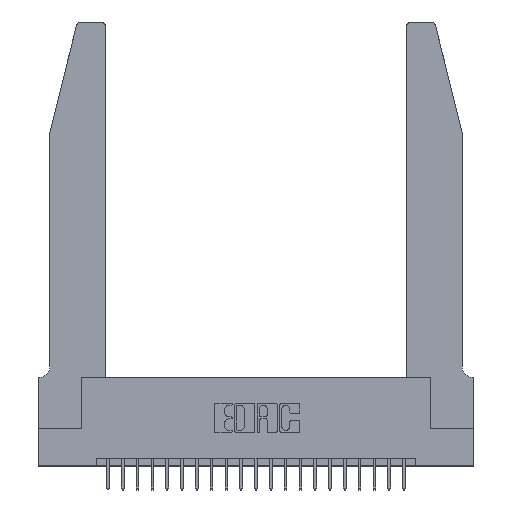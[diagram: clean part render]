
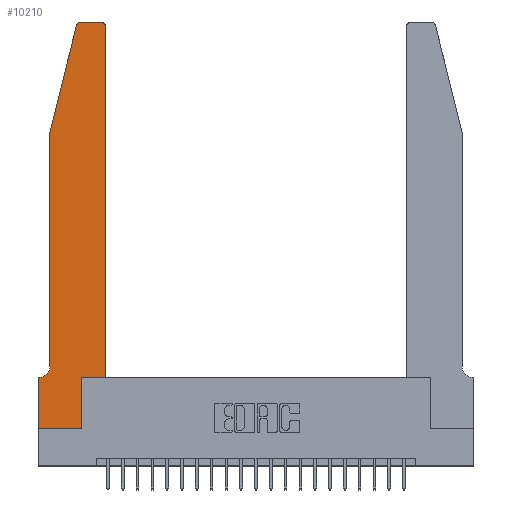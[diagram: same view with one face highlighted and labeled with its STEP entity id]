
A CAD part, top view. The second image highlights one B-rep face of the part: STEP entity #10210.
In plain terms, the highlighted planar face has unit normal (0, 0, 1).
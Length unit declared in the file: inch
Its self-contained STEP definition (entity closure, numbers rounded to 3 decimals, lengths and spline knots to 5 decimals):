
#518 = CARTESIAN_POINT ( 'NONE',  ( 0.4505, 0.35, 0.37 ) ) ;
#969 = ORIENTED_EDGE ( 'NONE', *, *, #10459, .T. ) ;
#1217 = CARTESIAN_POINT ( 'NONE',  ( 0.0755, 2., 0.37 ) ) ;
#1559 = LINE ( 'NONE', #3184, #14602 ) ;
#1598 = CARTESIAN_POINT ( 'NONE',  ( 0.284, 2.75, 0.37 ) ) ;
#2487 = EDGE_CURVE ( 'NONE', #15895, #18629, #21122, .T. ) ;
#2760 = DIRECTION ( 'NONE',  ( 0., -1., 0. ) ) ;
#3184 = CARTESIAN_POINT ( 'NONE',  ( 0.4505, 0.35, 0.37 ) ) ;
#3257 = EDGE_CURVE ( 'NONE', #16590, #14821, #1559, .T. ) ;
#3805 = AXIS2_PLACEMENT_3D ( 'NONE', #23059, #21273, #11658 ) ;
#3820 = VERTEX_POINT ( 'NONE', #13318 ) ;
#4041 = EDGE_CURVE ( 'NONE', #3820, #15895, #5825, .T. ) ;
#4322 = ORIENTED_EDGE ( 'NONE', *, *, #22397, .T. ) ;
#4391 = CIRCLE ( 'NONE', #15009, 0.03 ) ;
#4394 = DIRECTION ( 'NONE',  ( 0., 1., 0. ) ) ;
#4732 = CARTESIAN_POINT ( 'NONE',  ( 0., 0., 0.37 ) ) ;
#4847 = DIRECTION ( 'NONE',  ( -0.239, -0.971, 0. ) ) ;
#4970 = CARTESIAN_POINT ( 'NONE',  ( 0., 0.35, 0.37 ) ) ;
#5180 = ORIENTED_EDGE ( 'NONE', *, *, #2487, .T. ) ;
#5218 = CARTESIAN_POINT ( 'NONE',  ( 0.284, 2.72, 0.37 ) ) ;
#5219 = CARTESIAN_POINT ( 'NONE',  ( 0.2865, 0.35, 0.37 ) ) ;
#5332 = VERTEX_POINT ( 'NONE', #23850 ) ;
#5793 = CIRCLE ( 'NONE', #6472, 0.03 ) ;
#5825 = CIRCLE ( 'NONE', #21263, 0.07 ) ;
#6244 = PLANE ( 'NONE',  #3805 ) ;
#6345 = EDGE_CURVE ( 'NONE', #18629, #5332, #7026, .T. ) ;
#6351 = VERTEX_POINT ( 'NONE', #19138 ) ;
#6428 = EDGE_LOOP ( 'NONE', ( #13984, #10346, #16346, #15535, #10885, #5180, #6851, #6912, #17167, #21293, #969, #4322 ) ) ;
#6472 = AXIS2_PLACEMENT_3D ( 'NONE', #23549, #23231, #12160 ) ;
#6851 = ORIENTED_EDGE ( 'NONE', *, *, #6345, .T. ) ;
#6912 = ORIENTED_EDGE ( 'NONE', *, *, #23955, .T. ) ;
#7026 = LINE ( 'NONE', #11127, #11673 ) ;
#7093 = DIRECTION ( 'NONE',  ( 1., 0., 0. ) ) ;
#7565 = CARTESIAN_POINT ( 'NONE',  ( 0.0755, 0.35, 0.37 ) ) ;
#8272 = EDGE_CURVE ( 'NONE', #18080, #16590, #8691, .T. ) ;
#8353 = VECTOR ( 'NONE', #11817, 39.37008 ) ;
#8691 = LINE ( 'NONE', #14840, #23918 ) ;
#8903 = VERTEX_POINT ( 'NONE', #21593 ) ;
#9242 = VECTOR ( 'NONE', #18430, 39.37008 ) ;
#9879 = CARTESIAN_POINT ( 'NONE',  ( 0.4205, 2.75, 0.37 ) ) ;
#10094 = LINE ( 'NONE', #4732, #9242 ) ;
#10210 = ADVANCED_FACE ( 'NONE', ( #18243 ), #6244, .T. ) ;
#10346 = ORIENTED_EDGE ( 'NONE', *, *, #21312, .T. ) ;
#10459 = EDGE_CURVE ( 'NONE', #14821, #10575, #17035, .T. ) ;
#10575 = VERTEX_POINT ( 'NONE', #20795 ) ;
#10885 = ORIENTED_EDGE ( 'NONE', *, *, #4041, .T. ) ;
#11127 = CARTESIAN_POINT ( 'NONE',  ( 0., 0., 0.37 ) ) ;
#11249 = LINE ( 'NONE', #17401, #8353 ) ;
#11658 = DIRECTION ( 'NONE',  ( 1., 0., 0. ) ) ;
#11673 = VECTOR ( 'NONE', #2760, 39.37008 ) ;
#11817 = DIRECTION ( 'NONE',  ( -1., 0., 0. ) ) ;
#12160 = DIRECTION ( 'NONE',  ( 1., 0., 0. ) ) ;
#12227 = CARTESIAN_POINT ( 'NONE',  ( 0.2865, 0., 0.37 ) ) ;
#13318 = CARTESIAN_POINT ( 'NONE',  ( 0.0755, 0.42, 0.37 ) ) ;
#13984 = ORIENTED_EDGE ( 'NONE', *, *, #15101, .T. ) ;
#14243 = DIRECTION ( 'NONE',  ( 0., 1., 0. ) ) ;
#14574 = DIRECTION ( 'NONE',  ( 0., 0., 1. ) ) ;
#14602 = VECTOR ( 'NONE', #16005, 39.37008 ) ;
#14821 = VERTEX_POINT ( 'NONE', #20120 ) ;
#14840 = CARTESIAN_POINT ( 'NONE',  ( 0.2865, 0.35, 0.37 ) ) ;
#15009 = AXIS2_PLACEMENT_3D ( 'NONE', #5218, #14574, #7093 ) ;
#15010 = DIRECTION ( 'NONE',  ( -1., 0., 0. ) ) ;
#15101 = EDGE_CURVE ( 'NONE', #19637, #21372, #11249, .T. ) ;
#15158 = CARTESIAN_POINT ( 'NONE',  ( 0.0055, 0.42, 0.37 ) ) ;
#15535 = ORIENTED_EDGE ( 'NONE', *, *, #23777, .T. ) ;
#15895 = VERTEX_POINT ( 'NONE', #21940 ) ;
#16005 = DIRECTION ( 'NONE',  ( 1., 0., 0. ) ) ;
#16240 = VECTOR ( 'NONE', #22858, 39.37008 ) ;
#16346 = ORIENTED_EDGE ( 'NONE', *, *, #23406, .T. ) ;
#16590 = VERTEX_POINT ( 'NONE', #5219 ) ;
#17035 = LINE ( 'NONE', #518, #23518 ) ;
#17167 = ORIENTED_EDGE ( 'NONE', *, *, #8272, .T. ) ;
#17230 = DIRECTION ( 'NONE',  ( 0., 0., -1. ) ) ;
#17401 = CARTESIAN_POINT ( 'NONE',  ( 0.2605, 2.75, 0.37 ) ) ;
#17580 = VECTOR ( 'NONE', #21041, 39.37008 ) ;
#18080 = VERTEX_POINT ( 'NONE', #12227 ) ;
#18243 = FACE_OUTER_BOUND ( 'NONE', #6428, .T. ) ;
#18430 = DIRECTION ( 'NONE',  ( 1., 0., 0. ) ) ;
#18629 = VERTEX_POINT ( 'NONE', #4970 ) ;
#19105 = CARTESIAN_POINT ( 'NONE',  ( 0.0755, 2., 0.37 ) ) ;
#19138 = CARTESIAN_POINT ( 'NONE',  ( 0.25487, 2.72718, 0.37 ) ) ;
#19637 = VERTEX_POINT ( 'NONE', #9879 ) ;
#20120 = CARTESIAN_POINT ( 'NONE',  ( 0.4505, 0.35, 0.37 ) ) ;
#20795 = CARTESIAN_POINT ( 'NONE',  ( 0.4505, 2.72, 0.37 ) ) ;
#21041 = DIRECTION ( 'NONE',  ( -1., 0., 0. ) ) ;
#21122 = LINE ( 'NONE', #7565, #17580 ) ;
#21238 = LINE ( 'NONE', #19105, #16240 ) ;
#21263 = AXIS2_PLACEMENT_3D ( 'NONE', #15158, #17230, #15010 ) ;
#21273 = DIRECTION ( 'NONE',  ( 0., 0., 1. ) ) ;
#21293 = ORIENTED_EDGE ( 'NONE', *, *, #3257, .T. ) ;
#21312 = EDGE_CURVE ( 'NONE', #21372, #6351, #4391, .T. ) ;
#21372 = VERTEX_POINT ( 'NONE', #1598 ) ;
#21593 = CARTESIAN_POINT ( 'NONE',  ( 0.0755, 2., 0.37 ) ) ;
#21940 = CARTESIAN_POINT ( 'NONE',  ( 0.0055, 0.35, 0.37 ) ) ;
#22397 = EDGE_CURVE ( 'NONE', #10575, #19637, #5793, .T. ) ;
#22707 = LINE ( 'NONE', #1217, #23598 ) ;
#22858 = DIRECTION ( 'NONE',  ( 0., -1., 0. ) ) ;
#23059 = CARTESIAN_POINT ( 'NONE',  ( 0., 0.35, 0.37 ) ) ;
#23231 = DIRECTION ( 'NONE',  ( 0., 0., 1. ) ) ;
#23406 = EDGE_CURVE ( 'NONE', #6351, #8903, #22707, .T. ) ;
#23518 = VECTOR ( 'NONE', #4394, 39.37008 ) ;
#23549 = CARTESIAN_POINT ( 'NONE',  ( 0.4205, 2.72, 0.37 ) ) ;
#23598 = VECTOR ( 'NONE', #4847, 39.37008 ) ;
#23777 = EDGE_CURVE ( 'NONE', #8903, #3820, #21238, .T. ) ;
#23850 = CARTESIAN_POINT ( 'NONE',  ( 0., 0., 0.37 ) ) ;
#23918 = VECTOR ( 'NONE', #14243, 39.37008 ) ;
#23955 = EDGE_CURVE ( 'NONE', #5332, #18080, #10094, .T. ) ;
